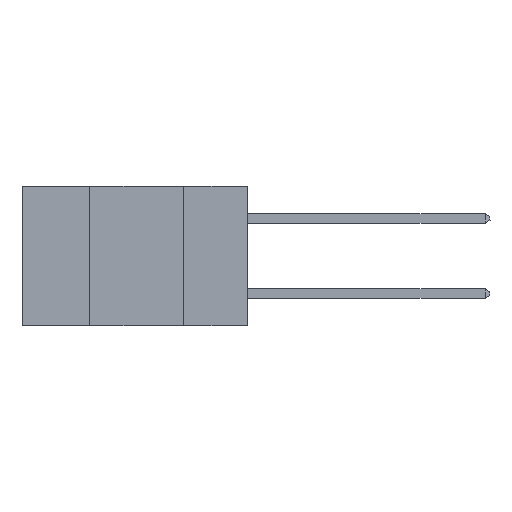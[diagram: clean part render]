
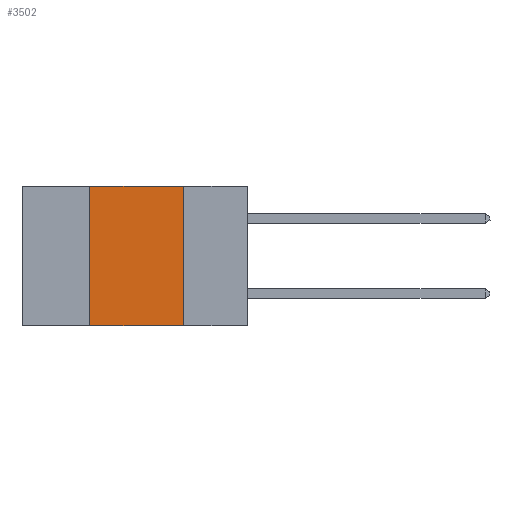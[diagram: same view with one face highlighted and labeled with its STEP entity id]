
A CAD part, left-side view. The second image highlights one B-rep face of the part: STEP entity #3502.
In plain terms, the highlighted planar face has unit normal (-1, 0, 0).
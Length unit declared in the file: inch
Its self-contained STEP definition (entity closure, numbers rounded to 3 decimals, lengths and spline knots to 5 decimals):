
#37 = EDGE_CURVE ( 'NONE', #10304, #8691, #1924, .T. ) ;
#617 = CARTESIAN_POINT ( 'NONE',  ( 0., 0.17, -0.37 ) ) ;
#624 = ORIENTED_EDGE ( 'NONE', *, *, #37, .F. ) ;
#1426 = EDGE_CURVE ( 'NONE', #10548, #1710, #2568, .T. ) ;
#1710 = VERTEX_POINT ( 'NONE', #8336 ) ;
#1924 = LINE ( 'NONE', #8352, #2182 ) ;
#2182 = VECTOR ( 'NONE', #7581, 39.37008 ) ;
#2292 = ORIENTED_EDGE ( 'NONE', *, *, #1426, .F. ) ;
#2335 = PLANE ( 'NONE',  #3060 ) ;
#2339 = CARTESIAN_POINT ( 'NONE',  ( 0., 0.42, 0. ) ) ;
#2568 = LINE ( 'NONE', #2339, #5886 ) ;
#3060 = AXIS2_PLACEMENT_3D ( 'NONE', #7299, #8125, #9017 ) ;
#3152 = VECTOR ( 'NONE', #3295, 39.37008 ) ;
#3169 = DIRECTION ( 'NONE',  ( 0., 0., 1. ) ) ;
#3295 = DIRECTION ( 'NONE',  ( 0., -1., 0. ) ) ;
#3502 = ADVANCED_FACE ( 'NONE', ( #5127 ), #2335, .F. ) ;
#4106 = CARTESIAN_POINT ( 'NONE',  ( 0., 0.6, 0. ) ) ;
#4288 = VECTOR ( 'NONE', #10063, 39.37008 ) ;
#4939 = LINE ( 'NONE', #4106, #3152 ) ;
#5048 = CARTESIAN_POINT ( 'NONE',  ( 0., 0.6, -0.37 ) ) ;
#5127 = FACE_OUTER_BOUND ( 'NONE', #10629, .T. ) ;
#5835 = EDGE_CURVE ( 'NONE', #1710, #10304, #4939, .T. ) ;
#5886 = VECTOR ( 'NONE', #3169, 39.37008 ) ;
#7299 = CARTESIAN_POINT ( 'NONE',  ( 0., 0.6, 0. ) ) ;
#7490 = CARTESIAN_POINT ( 'NONE',  ( 0., 0.17, 0. ) ) ;
#7548 = LINE ( 'NONE', #5048, #4288 ) ;
#7581 = DIRECTION ( 'NONE',  ( 0., 0., -1. ) ) ;
#8125 = DIRECTION ( 'NONE',  ( 1., 0., 0. ) ) ;
#8336 = CARTESIAN_POINT ( 'NONE',  ( 0., 0.42, 0. ) ) ;
#8352 = CARTESIAN_POINT ( 'NONE',  ( 0., 0.17, 0. ) ) ;
#8691 = VERTEX_POINT ( 'NONE', #617 ) ;
#9017 = DIRECTION ( 'NONE',  ( 0., 0., -1. ) ) ;
#9191 = ORIENTED_EDGE ( 'NONE', *, *, #10257, .T. ) ;
#10045 = CARTESIAN_POINT ( 'NONE',  ( 0., 0.42, -0.37 ) ) ;
#10063 = DIRECTION ( 'NONE',  ( 0., -1., 0. ) ) ;
#10257 = EDGE_CURVE ( 'NONE', #10548, #8691, #7548, .T. ) ;
#10304 = VERTEX_POINT ( 'NONE', #7490 ) ;
#10548 = VERTEX_POINT ( 'NONE', #10045 ) ;
#10629 = EDGE_LOOP ( 'NONE', ( #624, #10656, #2292, #9191 ) ) ;
#10656 = ORIENTED_EDGE ( 'NONE', *, *, #5835, .F. ) ;
